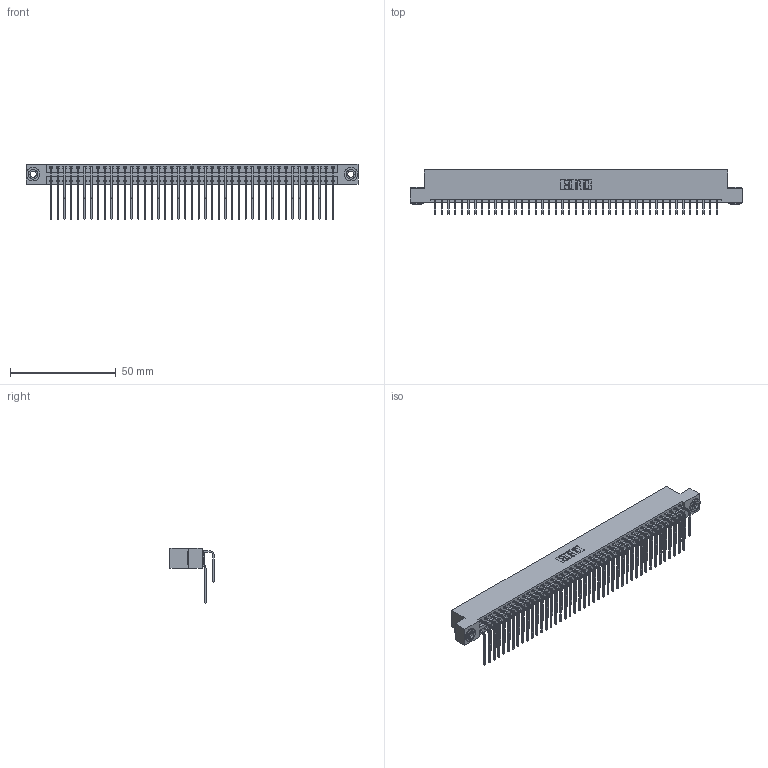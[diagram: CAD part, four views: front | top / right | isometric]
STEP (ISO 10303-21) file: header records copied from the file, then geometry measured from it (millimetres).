
FILE_DESCRIPTION (( 'STEP AP203' ), '1' );
FILE_NAME ('346-086-559-203.STEP', '2022-05-25T23:32:30', ( '' ), ( '' ), 'SwSTEP 2.0', 'SolidWorks 2020', '' );
FILE_SCHEMA (( 'CONFIG_CONTROL_DESIGN' ));
Length unit declared in the file: inch
Products named in the file (5): 346 Part_Flush Mounting Lugs - 0.156 Dia-TH; 346-086-559-203; 345-292-001_558 559 Tail - 1; 345-250-002_345-250-002-102; 345-292-001_559 Tail - 2
Assembly tree (89 placements, depth 2):
  346-086-559-203
    346 Part_Flush Mounting Lugs - 0.156 Dia-TH
    345-292-001_558 559 Tail - 1  x43
    345-292-001_559 Tail - 2  x43
    345-250-002_345-250-002-102  x2
Bounding box: 157.1 x 20.89 x 26.16 mm (x, y, z)
Volume: 15824.3 mm3; surface area: 24396 mm2
Topology: 89 solids, 89 shells, 4818 faces, 14287 edges, 9406 vertices
Faces by surface type: plane 3282, cylinder 1528, cone 8
Entity records: 30778 total; most frequent: CARTESIAN_POINT 5104, ORIENTED_EDGE 4978, DIRECTION 4551, EDGE_CURVE 2489, VECTOR 2121, LINE 2121, VERTEX_POINT 1654, AXIS2_PLACEMENT_3D 1215
